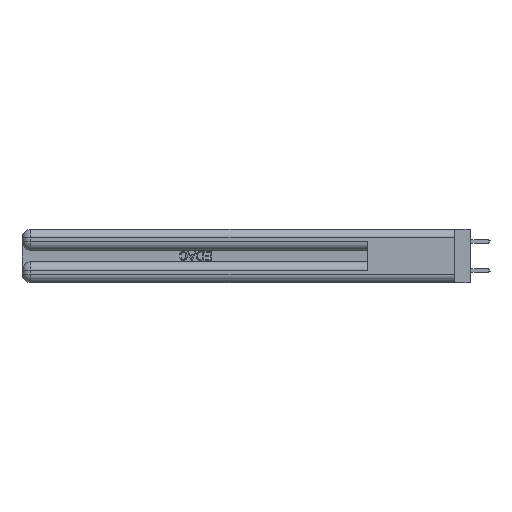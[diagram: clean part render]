
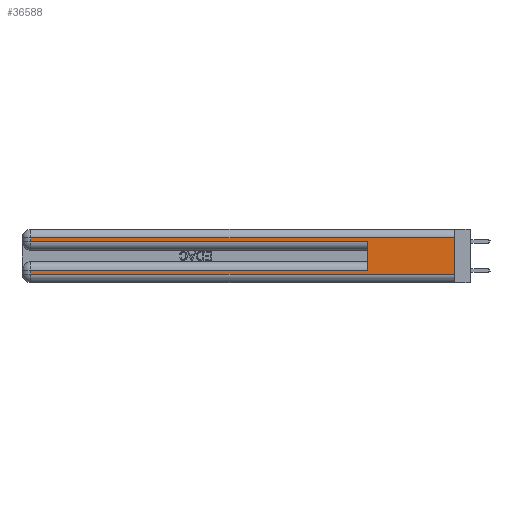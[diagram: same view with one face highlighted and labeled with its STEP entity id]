
A CAD part, left-side view. The second image highlights one B-rep face of the part: STEP entity #36588.
In plain terms, the highlighted planar face has unit normal (-1, 0, 0).
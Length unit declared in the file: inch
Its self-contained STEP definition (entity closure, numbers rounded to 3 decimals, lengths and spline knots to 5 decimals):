
#379 = ORIENTED_EDGE ( 'NONE', *, *, #12852, .F. ) ;
#1421 = ORIENTED_EDGE ( 'NONE', *, *, #26814, .T. ) ;
#1778 = EDGE_LOOP ( 'NONE', ( #23835, #2907, #39639, #23347, #379, #1421, #22841, #42194 ) ) ;
#2748 = VERTEX_POINT ( 'NONE', #6858 ) ;
#2907 = ORIENTED_EDGE ( 'NONE', *, *, #37155, .T. ) ;
#3044 = CARTESIAN_POINT ( 'NONE',  ( 0., 0.6, 0.145 ) ) ;
#4754 = FACE_OUTER_BOUND ( 'NONE', #1778, .T. ) ;
#6858 = CARTESIAN_POINT ( 'NONE',  ( 0., 0.6, 0.285 ) ) ;
#6888 = DIRECTION ( 'NONE',  ( 0., 0., -1. ) ) ;
#8459 = CARTESIAN_POINT ( 'NONE',  ( 0., 0., 0.37 ) ) ;
#8695 = DIRECTION ( 'NONE',  ( 0., 1., 0. ) ) ;
#9216 = EDGE_CURVE ( 'NONE', #23871, #13627, #35131, .T. ) ;
#11491 = CARTESIAN_POINT ( 'NONE',  ( 0., 2.94, 0.31 ) ) ;
#11717 = DIRECTION ( 'NONE',  ( 0., 0., -1. ) ) ;
#12506 = CARTESIAN_POINT ( 'NONE',  ( 0., 0., 0.06 ) ) ;
#12803 = CARTESIAN_POINT ( 'NONE',  ( 0., 0., 0.285 ) ) ;
#12852 = EDGE_CURVE ( 'NONE', #20369, #2748, #29226, .T. ) ;
#13627 = VERTEX_POINT ( 'NONE', #37059 ) ;
#13926 = EDGE_CURVE ( 'NONE', #26607, #13627, #31245, .T. ) ;
#14215 = DIRECTION ( 'NONE',  ( 0., 1., 0. ) ) ;
#14748 = EDGE_CURVE ( 'NONE', #18949, #26607, #35579, .T. ) ;
#15120 = CARTESIAN_POINT ( 'NONE',  ( 0., 0., 0.31 ) ) ;
#15276 = LINE ( 'NONE', #25964, #21926 ) ;
#16245 = DIRECTION ( 'NONE',  ( 0., 0., -1. ) ) ;
#17781 = VECTOR ( 'NONE', #14215, 39.37008 ) ;
#18949 = VERTEX_POINT ( 'NONE', #35839 ) ;
#20369 = VERTEX_POINT ( 'NONE', #37753 ) ;
#21926 = VECTOR ( 'NONE', #16245, 39.37008 ) ;
#22841 = ORIENTED_EDGE ( 'NONE', *, *, #14748, .T. ) ;
#23347 = ORIENTED_EDGE ( 'NONE', *, *, #34151, .T. ) ;
#23835 = ORIENTED_EDGE ( 'NONE', *, *, #9216, .F. ) ;
#23871 = VERTEX_POINT ( 'NONE', #26854 ) ;
#25609 = VECTOR ( 'NONE', #8695, 39.37008 ) ;
#25964 = CARTESIAN_POINT ( 'NONE',  ( 0., 2.94, 0.37 ) ) ;
#26241 = EDGE_CURVE ( 'NONE', #34571, #42114, #15276, .T. ) ;
#26432 = CARTESIAN_POINT ( 'NONE',  ( 0., 2.94, 0.37 ) ) ;
#26442 = LINE ( 'NONE', #36873, #17781 ) ;
#26607 = VERTEX_POINT ( 'NONE', #31191 ) ;
#26814 = EDGE_CURVE ( 'NONE', #20369, #18949, #26442, .T. ) ;
#26854 = CARTESIAN_POINT ( 'NONE',  ( 0., 0., 0.31 ) ) ;
#27410 = LINE ( 'NONE', #12803, #35007 ) ;
#28007 = PLANE ( 'NONE',  #38761 ) ;
#28142 = CARTESIAN_POINT ( 'NONE',  ( 0., 2.94, 0.285 ) ) ;
#29067 = DIRECTION ( 'NONE',  ( 0., -1., 0. ) ) ;
#29226 = LINE ( 'NONE', #3044, #36872 ) ;
#29663 = DIRECTION ( 'NONE',  ( 0., 0., -1. ) ) ;
#31191 = CARTESIAN_POINT ( 'NONE',  ( 0., 2.94, 0.06 ) ) ;
#31245 = LINE ( 'NONE', #12506, #40339 ) ;
#31263 = DIRECTION ( 'NONE',  ( 1., 0., 0. ) ) ;
#34125 = VECTOR ( 'NONE', #29663, 39.37008 ) ;
#34151 = EDGE_CURVE ( 'NONE', #42114, #2748, #27410, .T. ) ;
#34250 = LINE ( 'NONE', #15120, #25609 ) ;
#34571 = VERTEX_POINT ( 'NONE', #11491 ) ;
#34586 = VECTOR ( 'NONE', #6888, 39.37008 ) ;
#35007 = VECTOR ( 'NONE', #29067, 39.37008 ) ;
#35131 = LINE ( 'NONE', #39335, #34125 ) ;
#35298 = DIRECTION ( 'NONE',  ( 0., -1., 0. ) ) ;
#35579 = LINE ( 'NONE', #26432, #34586 ) ;
#35839 = CARTESIAN_POINT ( 'NONE',  ( 0., 2.94, 0.085 ) ) ;
#36588 = ADVANCED_FACE ( 'NONE', ( #4754 ), #28007, .F. ) ;
#36872 = VECTOR ( 'NONE', #38803, 39.37008 ) ;
#36873 = CARTESIAN_POINT ( 'NONE',  ( 0., 0., 0.085 ) ) ;
#37059 = CARTESIAN_POINT ( 'NONE',  ( 0., 0., 0.06 ) ) ;
#37155 = EDGE_CURVE ( 'NONE', #23871, #34571, #34250, .T. ) ;
#37753 = CARTESIAN_POINT ( 'NONE',  ( 0., 0.6, 0.085 ) ) ;
#38761 = AXIS2_PLACEMENT_3D ( 'NONE', #8459, #31263, #11717 ) ;
#38803 = DIRECTION ( 'NONE',  ( 0., 0., 1. ) ) ;
#39335 = CARTESIAN_POINT ( 'NONE',  ( 0., 0., 0.37 ) ) ;
#39639 = ORIENTED_EDGE ( 'NONE', *, *, #26241, .T. ) ;
#40339 = VECTOR ( 'NONE', #35298, 39.37008 ) ;
#42114 = VERTEX_POINT ( 'NONE', #28142 ) ;
#42194 = ORIENTED_EDGE ( 'NONE', *, *, #13926, .T. ) ;
